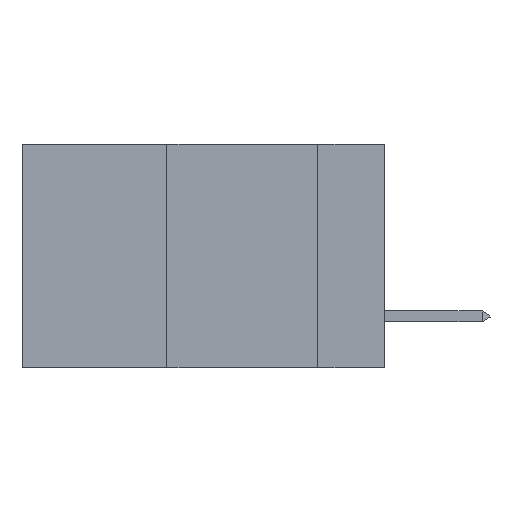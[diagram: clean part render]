
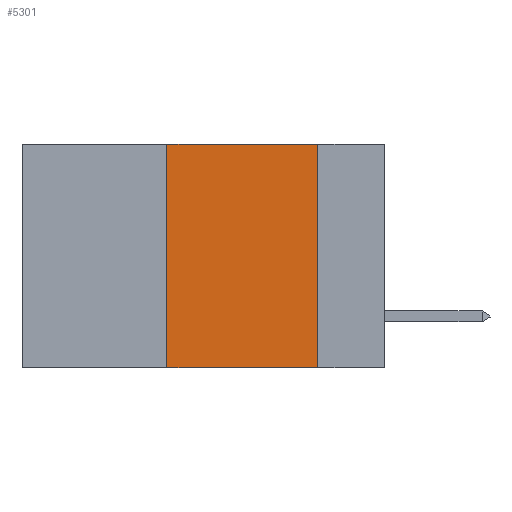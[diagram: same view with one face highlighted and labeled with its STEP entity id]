
A CAD part, left-side view. The second image highlights one B-rep face of the part: STEP entity #5301.
In plain terms, the highlighted planar face has unit normal (-1, 0, 0).
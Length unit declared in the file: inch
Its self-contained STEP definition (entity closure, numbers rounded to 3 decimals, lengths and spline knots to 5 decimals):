
#304 = CARTESIAN_POINT ( 'NONE',  ( 0., 0.6, -0.37 ) ) ;
#581 = VECTOR ( 'NONE', #4603, 39.37008 ) ;
#2289 = AXIS2_PLACEMENT_3D ( 'NONE', #9196, #6340, #15482 ) ;
#2543 = VERTEX_POINT ( 'NONE', #7954 ) ;
#2745 = EDGE_CURVE ( 'NONE', #15395, #2543, #10121, .T. ) ;
#3438 = LINE ( 'NONE', #304, #18503 ) ;
#4344 = EDGE_CURVE ( 'NONE', #16863, #15395, #4701, .T. ) ;
#4603 = DIRECTION ( 'NONE',  ( 0., 0., 1. ) ) ;
#4701 = LINE ( 'NONE', #10802, #581 ) ;
#4953 = EDGE_CURVE ( 'NONE', #2543, #13329, #13553, .T. ) ;
#5229 = EDGE_LOOP ( 'NONE', ( #7288, #10847, #11504, #14527 ) ) ;
#5301 = ADVANCED_FACE ( 'NONE', ( #8371 ), #13790, .F. ) ;
#6340 = DIRECTION ( 'NONE',  ( 1., 0., 0. ) ) ;
#7288 = ORIENTED_EDGE ( 'NONE', *, *, #4953, .F. ) ;
#7455 = CARTESIAN_POINT ( 'NONE',  ( 0., 0.36, -0.37 ) ) ;
#7634 = VECTOR ( 'NONE', #19984, 39.37008 ) ;
#7954 = CARTESIAN_POINT ( 'NONE',  ( 0., 0.11, 0. ) ) ;
#8330 = CARTESIAN_POINT ( 'NONE',  ( 0., 0.36, 0. ) ) ;
#8371 = FACE_OUTER_BOUND ( 'NONE', #5229, .T. ) ;
#9196 = CARTESIAN_POINT ( 'NONE',  ( 0., 0.6, 0. ) ) ;
#10121 = LINE ( 'NONE', #15057, #13803 ) ;
#10802 = CARTESIAN_POINT ( 'NONE',  ( 0., 0.36, 0. ) ) ;
#10847 = ORIENTED_EDGE ( 'NONE', *, *, #2745, .F. ) ;
#11180 = DIRECTION ( 'NONE',  ( 0., -1., 0. ) ) ;
#11504 = ORIENTED_EDGE ( 'NONE', *, *, #4344, .F. ) ;
#12474 = CARTESIAN_POINT ( 'NONE',  ( 0., 0.11, 0. ) ) ;
#12983 = CARTESIAN_POINT ( 'NONE',  ( 0., 0.11, -0.37 ) ) ;
#13329 = VERTEX_POINT ( 'NONE', #12983 ) ;
#13553 = LINE ( 'NONE', #12474, #7634 ) ;
#13790 = PLANE ( 'NONE',  #2289 ) ;
#13803 = VECTOR ( 'NONE', #19760, 39.37008 ) ;
#14527 = ORIENTED_EDGE ( 'NONE', *, *, #16449, .T. ) ;
#15057 = CARTESIAN_POINT ( 'NONE',  ( 0., 0.6, 0. ) ) ;
#15395 = VERTEX_POINT ( 'NONE', #8330 ) ;
#15482 = DIRECTION ( 'NONE',  ( 0., 0., -1. ) ) ;
#16449 = EDGE_CURVE ( 'NONE', #16863, #13329, #3438, .T. ) ;
#16863 = VERTEX_POINT ( 'NONE', #7455 ) ;
#18503 = VECTOR ( 'NONE', #11180, 39.37008 ) ;
#19760 = DIRECTION ( 'NONE',  ( 0., -1., 0. ) ) ;
#19984 = DIRECTION ( 'NONE',  ( 0., 0., -1. ) ) ;
